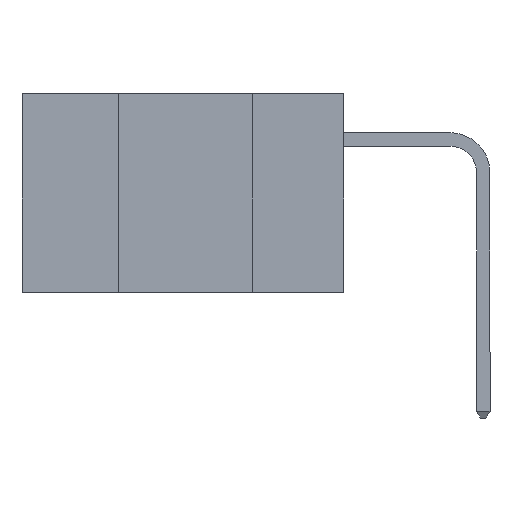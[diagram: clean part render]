
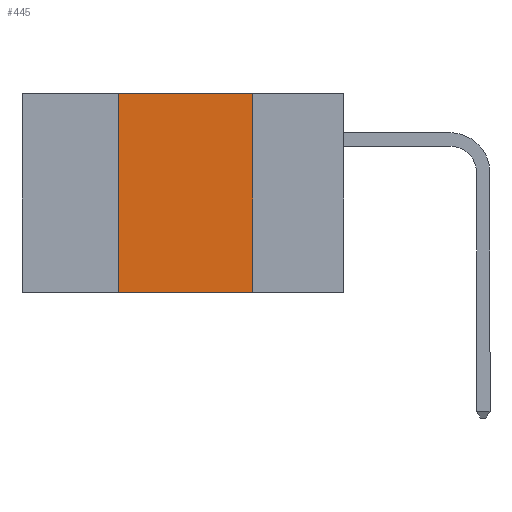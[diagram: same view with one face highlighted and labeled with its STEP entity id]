
A CAD part, left-side view. The second image highlights one B-rep face of the part: STEP entity #445.
In plain terms, the highlighted planar face has unit normal (-1, 0, 0).
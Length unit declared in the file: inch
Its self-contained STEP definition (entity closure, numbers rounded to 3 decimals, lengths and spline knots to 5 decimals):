
#115 = DIRECTION ( 'NONE',  ( 0., -1., 0. ) ) ;
#186 = CARTESIAN_POINT ( 'NONE',  ( 0., 0.42, -0.37 ) ) ;
#421 = LINE ( 'NONE', #3437, #2804 ) ;
#445 = ADVANCED_FACE ( 'NONE', ( #7271 ), #3207, .F. ) ;
#623 = DIRECTION ( 'NONE',  ( 0., 0., -1. ) ) ;
#698 = DIRECTION ( 'NONE',  ( 1., 0., 0. ) ) ;
#923 = EDGE_CURVE ( 'NONE', #4869, #3161, #2392, .T. ) ;
#935 = VERTEX_POINT ( 'NONE', #2435 ) ;
#1291 = EDGE_LOOP ( 'NONE', ( #4723, #1326, #2299, #2548 ) ) ;
#1326 = ORIENTED_EDGE ( 'NONE', *, *, #4788, .F. ) ;
#1408 = LINE ( 'NONE', #4080, #6081 ) ;
#2299 = ORIENTED_EDGE ( 'NONE', *, *, #923, .F. ) ;
#2392 = LINE ( 'NONE', #3769, #4268 ) ;
#2435 = CARTESIAN_POINT ( 'NONE',  ( 0., 0.17, 0. ) ) ;
#2548 = ORIENTED_EDGE ( 'NONE', *, *, #4307, .T. ) ;
#2804 = VECTOR ( 'NONE', #115, 39.37008 ) ;
#2889 = CARTESIAN_POINT ( 'NONE',  ( 0., 0.6, 0. ) ) ;
#3161 = VERTEX_POINT ( 'NONE', #5852 ) ;
#3207 = PLANE ( 'NONE',  #7152 ) ;
#3437 = CARTESIAN_POINT ( 'NONE',  ( 0., 0.6, -0.37 ) ) ;
#3769 = CARTESIAN_POINT ( 'NONE',  ( 0., 0.42, -0.37 ) ) ;
#4080 = CARTESIAN_POINT ( 'NONE',  ( 0., 0.17, -0.37 ) ) ;
#4268 = VECTOR ( 'NONE', #7738, 39.37008 ) ;
#4307 = EDGE_CURVE ( 'NONE', #4869, #8114, #421, .T. ) ;
#4348 = VECTOR ( 'NONE', #6776, 39.37008 ) ;
#4723 = ORIENTED_EDGE ( 'NONE', *, *, #6138, .F. ) ;
#4788 = EDGE_CURVE ( 'NONE', #3161, #935, #7534, .T. ) ;
#4869 = VERTEX_POINT ( 'NONE', #186 ) ;
#5841 = CARTESIAN_POINT ( 'NONE',  ( 0., 0.6, 0. ) ) ;
#5852 = CARTESIAN_POINT ( 'NONE',  ( 0., 0.42, 0. ) ) ;
#6081 = VECTOR ( 'NONE', #6682, 39.37008 ) ;
#6138 = EDGE_CURVE ( 'NONE', #935, #8114, #1408, .T. ) ;
#6682 = DIRECTION ( 'NONE',  ( 0., 0., -1. ) ) ;
#6776 = DIRECTION ( 'NONE',  ( 0., -1., 0. ) ) ;
#7135 = CARTESIAN_POINT ( 'NONE',  ( 0., 0.17, -0.37 ) ) ;
#7152 = AXIS2_PLACEMENT_3D ( 'NONE', #5841, #698, #623 ) ;
#7271 = FACE_OUTER_BOUND ( 'NONE', #1291, .T. ) ;
#7534 = LINE ( 'NONE', #2889, #4348 ) ;
#7738 = DIRECTION ( 'NONE',  ( 0., 0., 1. ) ) ;
#8114 = VERTEX_POINT ( 'NONE', #7135 ) ;
